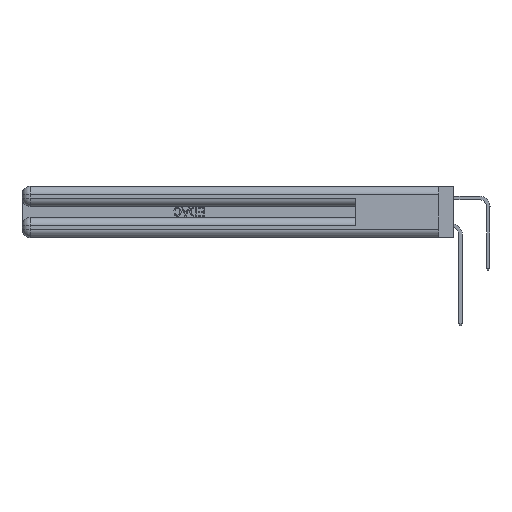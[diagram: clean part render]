
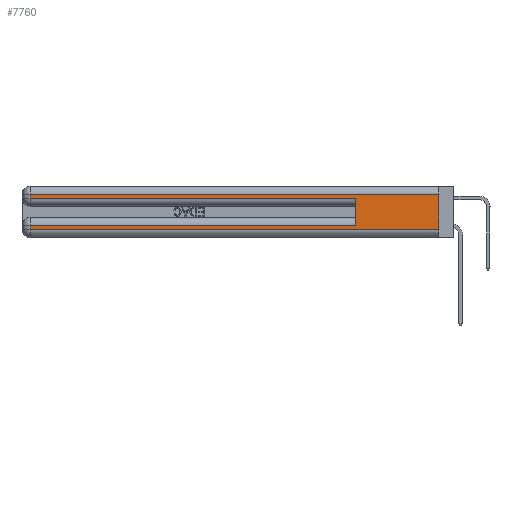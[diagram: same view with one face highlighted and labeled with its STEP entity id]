
A CAD part, left-side view. The second image highlights one B-rep face of the part: STEP entity #7760.
In plain terms, the highlighted planar face has unit normal (-1, 0, 0).
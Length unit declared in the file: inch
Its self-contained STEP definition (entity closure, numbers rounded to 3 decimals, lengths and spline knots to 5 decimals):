
#1913 = LINE ( 'NONE', #32162, #10552 ) ;
#2674 = CARTESIAN_POINT ( 'NONE',  ( 0., 0.6, 0.145 ) ) ;
#2717 = VECTOR ( 'NONE', #17936, 39.37008 ) ;
#3546 = VECTOR ( 'NONE', #22121, 39.37008 ) ;
#4297 = ORIENTED_EDGE ( 'NONE', *, *, #20355, .F. ) ;
#4401 = DIRECTION ( 'NONE',  ( 0., 0., -1. ) ) ;
#4523 = EDGE_CURVE ( 'NONE', #32387, #37922, #23960, .T. ) ;
#4586 = ORIENTED_EDGE ( 'NONE', *, *, #34640, .T. ) ;
#5367 = VERTEX_POINT ( 'NONE', #36284 ) ;
#5888 = EDGE_CURVE ( 'NONE', #40842, #20159, #26331, .T. ) ;
#6773 = CARTESIAN_POINT ( 'NONE',  ( 0., 2.94, 0.285 ) ) ;
#7760 = ADVANCED_FACE ( 'NONE', ( #20711 ), #40302, .F. ) ;
#8619 = CARTESIAN_POINT ( 'NONE',  ( 0., 2.94, 0.06 ) ) ;
#9486 = AXIS2_PLACEMENT_3D ( 'NONE', #10995, #44806, #36639 ) ;
#9857 = DIRECTION ( 'NONE',  ( 0., -1., 0. ) ) ;
#10552 = VECTOR ( 'NONE', #18542, 39.37008 ) ;
#10995 = CARTESIAN_POINT ( 'NONE',  ( 0., 0., 0.37 ) ) ;
#11558 = CARTESIAN_POINT ( 'NONE',  ( 0., 0., 0.085 ) ) ;
#13404 = LINE ( 'NONE', #43438, #16664 ) ;
#13969 = CARTESIAN_POINT ( 'NONE',  ( 0., 2.94, 0.085 ) ) ;
#15543 = ORIENTED_EDGE ( 'NONE', *, *, #35509, .F. ) ;
#16062 = LINE ( 'NONE', #26963, #24266 ) ;
#16664 = VECTOR ( 'NONE', #4401, 39.37008 ) ;
#16974 = DIRECTION ( 'NONE',  ( 0., 0., -1. ) ) ;
#17936 = DIRECTION ( 'NONE',  ( 0., -1., 0. ) ) ;
#18346 = ORIENTED_EDGE ( 'NONE', *, *, #4523, .T. ) ;
#18542 = DIRECTION ( 'NONE',  ( 0., 0., -1. ) ) ;
#20159 = VERTEX_POINT ( 'NONE', #26551 ) ;
#20355 = EDGE_CURVE ( 'NONE', #5367, #37922, #31486, .T. ) ;
#20711 = FACE_OUTER_BOUND ( 'NONE', #40011, .T. ) ;
#21636 = EDGE_CURVE ( 'NONE', #5367, #28670, #39500, .T. ) ;
#22121 = DIRECTION ( 'NONE',  ( 0., 1., 0. ) ) ;
#23229 = ORIENTED_EDGE ( 'NONE', *, *, #33897, .T. ) ;
#23763 = ORIENTED_EDGE ( 'NONE', *, *, #5888, .T. ) ;
#23960 = LINE ( 'NONE', #27654, #2717 ) ;
#24266 = VECTOR ( 'NONE', #16974, 39.37008 ) ;
#24947 = VERTEX_POINT ( 'NONE', #8619 ) ;
#26331 = LINE ( 'NONE', #36517, #37172 ) ;
#26551 = CARTESIAN_POINT ( 'NONE',  ( 0., 2.94, 0.31 ) ) ;
#26963 = CARTESIAN_POINT ( 'NONE',  ( 0., 2.94, 0.37 ) ) ;
#27436 = ORIENTED_EDGE ( 'NONE', *, *, #21636, .T. ) ;
#27654 = CARTESIAN_POINT ( 'NONE',  ( 0., 0., 0.285 ) ) ;
#28670 = VERTEX_POINT ( 'NONE', #13969 ) ;
#29942 = VECTOR ( 'NONE', #9857, 39.37008 ) ;
#30499 = CARTESIAN_POINT ( 'NONE',  ( 0., 0., 0.06 ) ) ;
#31486 = LINE ( 'NONE', #2674, #35807 ) ;
#32162 = CARTESIAN_POINT ( 'NONE',  ( 0., 0., 0.37 ) ) ;
#32387 = VERTEX_POINT ( 'NONE', #6773 ) ;
#32604 = LINE ( 'NONE', #30499, #29942 ) ;
#33897 = EDGE_CURVE ( 'NONE', #28670, #24947, #13404, .T. ) ;
#34640 = EDGE_CURVE ( 'NONE', #20159, #32387, #16062, .T. ) ;
#34943 = CARTESIAN_POINT ( 'NONE',  ( 0., 0., 0.31 ) ) ;
#35509 = EDGE_CURVE ( 'NONE', #40842, #35749, #1913, .T. ) ;
#35749 = VERTEX_POINT ( 'NONE', #44683 ) ;
#35807 = VECTOR ( 'NONE', #40404, 39.37008 ) ;
#36284 = CARTESIAN_POINT ( 'NONE',  ( 0., 0.6, 0.085 ) ) ;
#36443 = CARTESIAN_POINT ( 'NONE',  ( 0., 0.6, 0.285 ) ) ;
#36517 = CARTESIAN_POINT ( 'NONE',  ( 0., 0., 0.31 ) ) ;
#36639 = DIRECTION ( 'NONE',  ( 0., 0., -1. ) ) ;
#37172 = VECTOR ( 'NONE', #43534, 39.37008 ) ;
#37922 = VERTEX_POINT ( 'NONE', #36443 ) ;
#39500 = LINE ( 'NONE', #11558, #3546 ) ;
#40011 = EDGE_LOOP ( 'NONE', ( #15543, #23763, #4586, #18346, #4297, #27436, #23229, #42491 ) ) ;
#40302 = PLANE ( 'NONE',  #9486 ) ;
#40404 = DIRECTION ( 'NONE',  ( 0., 0., 1. ) ) ;
#40842 = VERTEX_POINT ( 'NONE', #34943 ) ;
#42491 = ORIENTED_EDGE ( 'NONE', *, *, #43972, .T. ) ;
#43438 = CARTESIAN_POINT ( 'NONE',  ( 0., 2.94, 0.37 ) ) ;
#43534 = DIRECTION ( 'NONE',  ( 0., 1., 0. ) ) ;
#43972 = EDGE_CURVE ( 'NONE', #24947, #35749, #32604, .T. ) ;
#44683 = CARTESIAN_POINT ( 'NONE',  ( 0., 0., 0.06 ) ) ;
#44806 = DIRECTION ( 'NONE',  ( 1., 0., 0. ) ) ;
